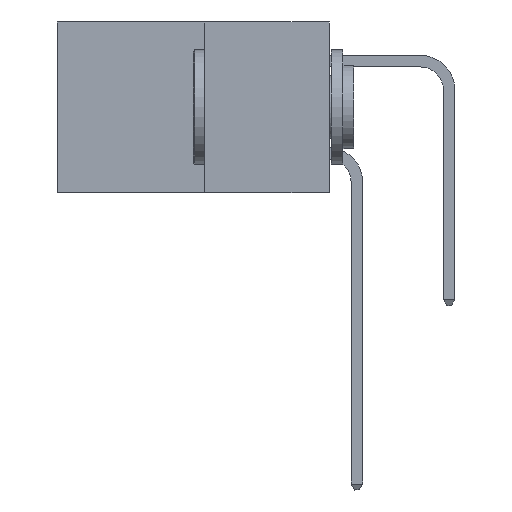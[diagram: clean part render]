
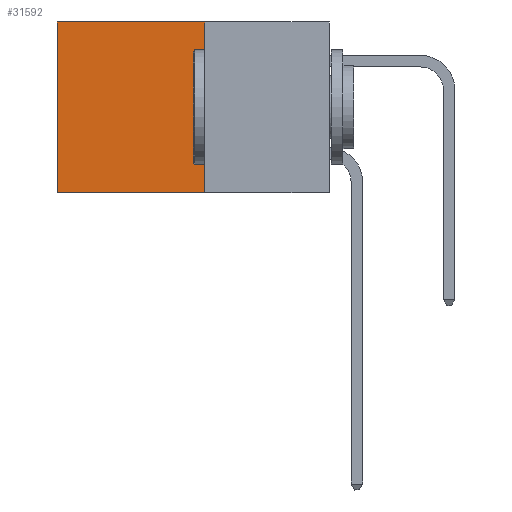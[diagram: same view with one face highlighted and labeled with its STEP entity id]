
A CAD part, left-side view. The second image highlights one B-rep face of the part: STEP entity #31592.
In plain terms, the highlighted planar face has unit normal (-1, 0, 0).
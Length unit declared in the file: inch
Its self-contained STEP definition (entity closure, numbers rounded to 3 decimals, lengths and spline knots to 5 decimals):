
#1322 = VERTEX_POINT ( 'NONE', #7902 ) ;
#2829 = VECTOR ( 'NONE', #26594, 39.37008 ) ;
#3538 = DIRECTION ( 'NONE',  ( 0., 0., -1. ) ) ;
#3650 = CARTESIAN_POINT ( 'NONE',  ( 0.277, 0.59, -0.37 ) ) ;
#5207 = EDGE_CURVE ( 'NONE', #1322, #19356, #15622, .T. ) ;
#5563 = FACE_OUTER_BOUND ( 'NONE', #33634, .T. ) ;
#6976 = VERTEX_POINT ( 'NONE', #32574 ) ;
#7274 = ORIENTED_EDGE ( 'NONE', *, *, #24447, .F. ) ;
#7902 = CARTESIAN_POINT ( 'NONE',  ( 0.277, 0.59, 0. ) ) ;
#7940 = CARTESIAN_POINT ( 'NONE',  ( 0.277, 0.27, -0.37 ) ) ;
#10664 = DIRECTION ( 'NONE',  ( 0., 0., -1. ) ) ;
#11502 = ORIENTED_EDGE ( 'NONE', *, *, #26024, .T. ) ;
#13247 = PLANE ( 'NONE',  #31501 ) ;
#13844 = DIRECTION ( 'NONE',  ( 0., 1., 0. ) ) ;
#15622 = LINE ( 'NONE', #3650, #22776 ) ;
#16490 = VECTOR ( 'NONE', #23850, 39.37008 ) ;
#17545 = VECTOR ( 'NONE', #13844, 39.37008 ) ;
#18099 = ORIENTED_EDGE ( 'NONE', *, *, #33226, .F. ) ;
#19356 = VERTEX_POINT ( 'NONE', #27732 ) ;
#22776 = VECTOR ( 'NONE', #3538, 39.37008 ) ;
#23664 = LINE ( 'NONE', #34596, #16490 ) ;
#23823 = CARTESIAN_POINT ( 'NONE',  ( 0.277, 0.27, -0.37 ) ) ;
#23850 = DIRECTION ( 'NONE',  ( 0., 0., -1. ) ) ;
#24439 = LINE ( 'NONE', #23823, #2829 ) ;
#24447 = EDGE_CURVE ( 'NONE', #6976, #19356, #24439, .T. ) ;
#24962 = VERTEX_POINT ( 'NONE', #26221 ) ;
#25618 = LINE ( 'NONE', #27342, #17545 ) ;
#26024 = EDGE_CURVE ( 'NONE', #24962, #1322, #25618, .T. ) ;
#26221 = CARTESIAN_POINT ( 'NONE',  ( 0.277, 0.27, 0. ) ) ;
#26594 = DIRECTION ( 'NONE',  ( 0., 1., 0. ) ) ;
#26870 = DIRECTION ( 'NONE',  ( 1., 0., 0. ) ) ;
#27342 = CARTESIAN_POINT ( 'NONE',  ( 0.277, 0.27, 0. ) ) ;
#27732 = CARTESIAN_POINT ( 'NONE',  ( 0.277, 0.59, -0.37 ) ) ;
#30309 = ORIENTED_EDGE ( 'NONE', *, *, #5207, .T. ) ;
#31501 = AXIS2_PLACEMENT_3D ( 'NONE', #7940, #26870, #10664 ) ;
#31592 = ADVANCED_FACE ( 'NONE', ( #5563 ), #13247, .F. ) ;
#32574 = CARTESIAN_POINT ( 'NONE',  ( 0.277, 0.27, -0.37 ) ) ;
#33226 = EDGE_CURVE ( 'NONE', #24962, #6976, #23664, .T. ) ;
#33634 = EDGE_LOOP ( 'NONE', ( #30309, #7274, #18099, #11502 ) ) ;
#34596 = CARTESIAN_POINT ( 'NONE',  ( 0.277, 0.27, -0.37 ) ) ;
